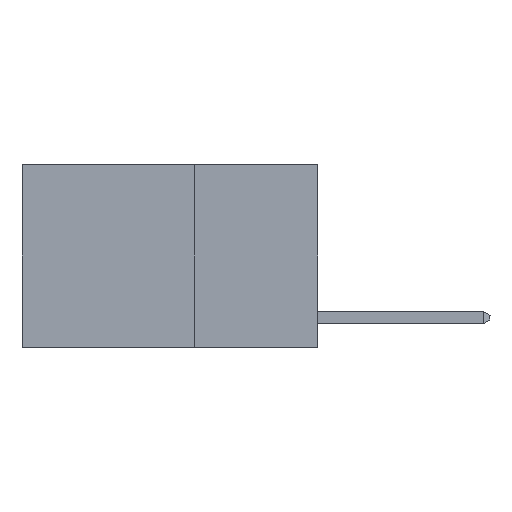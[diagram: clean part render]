
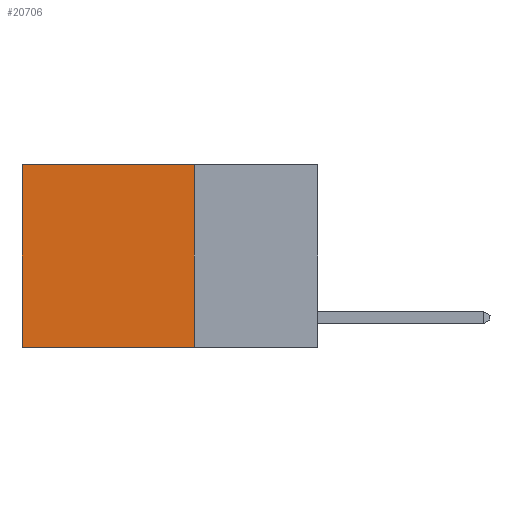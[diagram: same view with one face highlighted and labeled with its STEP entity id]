
A CAD part, left-side view. The second image highlights one B-rep face of the part: STEP entity #20706.
In plain terms, the highlighted planar face has unit normal (-1, 0, 0).
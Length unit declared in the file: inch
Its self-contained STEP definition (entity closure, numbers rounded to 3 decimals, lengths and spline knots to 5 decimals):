
#323 = EDGE_LOOP ( 'NONE', ( #4936, #16621, #24927, #21734 ) ) ;
#2474 = CARTESIAN_POINT ( 'NONE',  ( 0.2625, 0.25, 0. ) ) ;
#2828 = DIRECTION ( 'NONE',  ( 0., 0., -1. ) ) ;
#2862 = DIRECTION ( 'NONE',  ( 0., 0., -1. ) ) ;
#2913 = CARTESIAN_POINT ( 'NONE',  ( 0.2625, 0.25, 0. ) ) ;
#4714 = DIRECTION ( 'NONE',  ( 0., 1., 0. ) ) ;
#4936 = ORIENTED_EDGE ( 'NONE', *, *, #26406, .T. ) ;
#5628 = VECTOR ( 'NONE', #7064, 39.37008 ) ;
#6073 = VERTEX_POINT ( 'NONE', #24490 ) ;
#6107 = CARTESIAN_POINT ( 'NONE',  ( 0.2625, 0.25, 0. ) ) ;
#6729 = LINE ( 'NONE', #13023, #23590 ) ;
#7064 = DIRECTION ( 'NONE',  ( 0., 0., -1. ) ) ;
#7568 = VECTOR ( 'NONE', #13921, 39.37008 ) ;
#8050 = EDGE_CURVE ( 'NONE', #25345, #9772, #25943, .T. ) ;
#9772 = VERTEX_POINT ( 'NONE', #17830 ) ;
#9850 = LINE ( 'NONE', #11395, #7568 ) ;
#11334 = AXIS2_PLACEMENT_3D ( 'NONE', #24085, #25003, #2862 ) ;
#11395 = CARTESIAN_POINT ( 'NONE',  ( 0.2625, 0.25, -0.37 ) ) ;
#12514 = VECTOR ( 'NONE', #4714, 39.37008 ) ;
#13023 = CARTESIAN_POINT ( 'NONE',  ( 0.2625, 0.6, 0. ) ) ;
#13921 = DIRECTION ( 'NONE',  ( 0., 1., 0. ) ) ;
#16621 = ORIENTED_EDGE ( 'NONE', *, *, #26998, .F. ) ;
#17669 = VERTEX_POINT ( 'NONE', #26795 ) ;
#17807 = PLANE ( 'NONE',  #11334 ) ;
#17830 = CARTESIAN_POINT ( 'NONE',  ( 0.2625, 0.6, 0. ) ) ;
#19756 = LINE ( 'NONE', #2474, #5628 ) ;
#20706 = ADVANCED_FACE ( 'NONE', ( #27104 ), #17807, .F. ) ;
#21734 = ORIENTED_EDGE ( 'NONE', *, *, #8050, .T. ) ;
#23590 = VECTOR ( 'NONE', #2828, 39.37008 ) ;
#23689 = EDGE_CURVE ( 'NONE', #25345, #17669, #19756, .T. ) ;
#24085 = CARTESIAN_POINT ( 'NONE',  ( 0.2625, 0.25, 0. ) ) ;
#24490 = CARTESIAN_POINT ( 'NONE',  ( 0.2625, 0.6, -0.37 ) ) ;
#24927 = ORIENTED_EDGE ( 'NONE', *, *, #23689, .F. ) ;
#25003 = DIRECTION ( 'NONE',  ( 1., 0., 0. ) ) ;
#25345 = VERTEX_POINT ( 'NONE', #6107 ) ;
#25943 = LINE ( 'NONE', #2913, #12514 ) ;
#26406 = EDGE_CURVE ( 'NONE', #9772, #6073, #6729, .T. ) ;
#26795 = CARTESIAN_POINT ( 'NONE',  ( 0.2625, 0.25, -0.37 ) ) ;
#26998 = EDGE_CURVE ( 'NONE', #17669, #6073, #9850, .T. ) ;
#27104 = FACE_OUTER_BOUND ( 'NONE', #323, .T. ) ;
